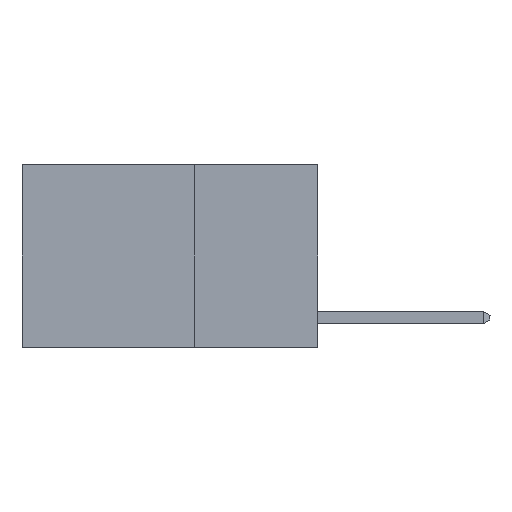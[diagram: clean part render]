
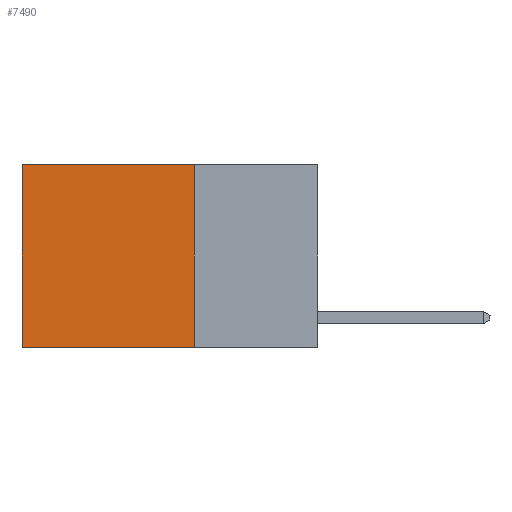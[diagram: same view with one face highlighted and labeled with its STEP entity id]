
A CAD part, left-side view. The second image highlights one B-rep face of the part: STEP entity #7490.
In plain terms, the highlighted planar face has unit normal (-1, 0, 0).
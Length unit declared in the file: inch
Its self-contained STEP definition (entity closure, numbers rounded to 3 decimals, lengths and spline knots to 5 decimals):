
#84 = VERTEX_POINT ( 'NONE', #8090 ) ;
#170 = ORIENTED_EDGE ( 'NONE', *, *, #3586, .T. ) ;
#286 = EDGE_CURVE ( 'NONE', #84, #12058, #5128, .T. ) ;
#1091 = AXIS2_PLACEMENT_3D ( 'NONE', #12947, #14098, #15209 ) ;
#1566 = CARTESIAN_POINT ( 'NONE',  ( 0.2625, 0.25, 0. ) ) ;
#3035 = EDGE_CURVE ( 'NONE', #15877, #13249, #3629, .T. ) ;
#3586 = EDGE_CURVE ( 'NONE', #13249, #12058, #11646, .T. ) ;
#3629 = LINE ( 'NONE', #5054, #15873 ) ;
#3998 = DIRECTION ( 'NONE',  ( 0., 0., -1. ) ) ;
#5054 = CARTESIAN_POINT ( 'NONE',  ( 0.2625, 0.25, 0. ) ) ;
#5110 = CARTESIAN_POINT ( 'NONE',  ( 0.2625, 0.6, 0. ) ) ;
#5128 = LINE ( 'NONE', #13826, #13063 ) ;
#5249 = FACE_OUTER_BOUND ( 'NONE', #6300, .T. ) ;
#5292 = DIRECTION ( 'NONE',  ( 0., 1., 0. ) ) ;
#6300 = EDGE_LOOP ( 'NONE', ( #170, #8353, #15255, #8252 ) ) ;
#6739 = EDGE_CURVE ( 'NONE', #15877, #84, #14717, .T. ) ;
#7490 = ADVANCED_FACE ( 'NONE', ( #5249 ), #13866, .F. ) ;
#7924 = VECTOR ( 'NONE', #14630, 39.37008 ) ;
#7958 = CARTESIAN_POINT ( 'NONE',  ( 0.2625, 0.6, 0. ) ) ;
#8090 = CARTESIAN_POINT ( 'NONE',  ( 0.2625, 0.25, -0.37 ) ) ;
#8252 = ORIENTED_EDGE ( 'NONE', *, *, #3035, .T. ) ;
#8353 = ORIENTED_EDGE ( 'NONE', *, *, #286, .F. ) ;
#11646 = LINE ( 'NONE', #7958, #12218 ) ;
#12058 = VERTEX_POINT ( 'NONE', #15224 ) ;
#12087 = CARTESIAN_POINT ( 'NONE',  ( 0.2625, 0.25, 0. ) ) ;
#12218 = VECTOR ( 'NONE', #3998, 39.37008 ) ;
#12266 = DIRECTION ( 'NONE',  ( 0., 1., 0. ) ) ;
#12947 = CARTESIAN_POINT ( 'NONE',  ( 0.2625, 0.25, 0. ) ) ;
#13063 = VECTOR ( 'NONE', #5292, 39.37008 ) ;
#13249 = VERTEX_POINT ( 'NONE', #5110 ) ;
#13826 = CARTESIAN_POINT ( 'NONE',  ( 0.2625, 0.25, -0.37 ) ) ;
#13866 = PLANE ( 'NONE',  #1091 ) ;
#14098 = DIRECTION ( 'NONE',  ( 1., 0., 0. ) ) ;
#14630 = DIRECTION ( 'NONE',  ( 0., 0., -1. ) ) ;
#14717 = LINE ( 'NONE', #12087, #7924 ) ;
#15209 = DIRECTION ( 'NONE',  ( 0., 0., -1. ) ) ;
#15224 = CARTESIAN_POINT ( 'NONE',  ( 0.2625, 0.6, -0.37 ) ) ;
#15255 = ORIENTED_EDGE ( 'NONE', *, *, #6739, .F. ) ;
#15873 = VECTOR ( 'NONE', #12266, 39.37008 ) ;
#15877 = VERTEX_POINT ( 'NONE', #1566 ) ;
